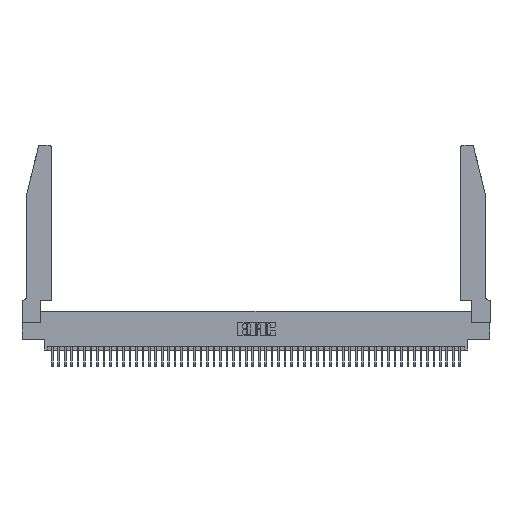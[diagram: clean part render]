
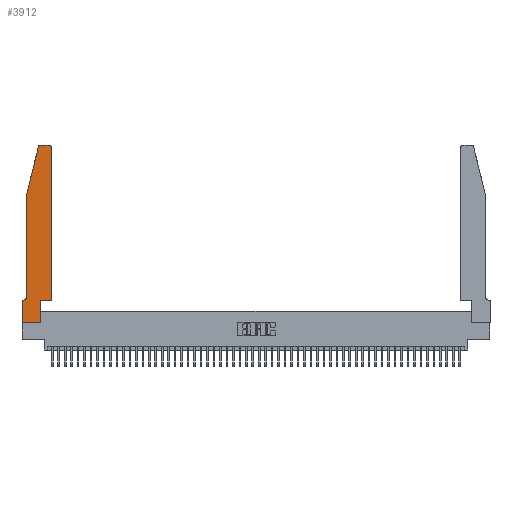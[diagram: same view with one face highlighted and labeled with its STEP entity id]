
A CAD part, top view. The second image highlights one B-rep face of the part: STEP entity #3912.
In plain terms, the highlighted planar face has unit normal (0, 0, 1).
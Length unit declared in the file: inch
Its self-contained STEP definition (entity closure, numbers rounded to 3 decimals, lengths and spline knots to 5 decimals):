
#537 = DIRECTION ( 'NONE',  ( 0., 0., 1. ) ) ;
#1796 = CARTESIAN_POINT ( 'NONE',  ( 0.4505, 0.35, 0.37 ) ) ;
#2151 = EDGE_CURVE ( 'NONE', #37562, #42521, #5699, .T. ) ;
#2193 = LINE ( 'NONE', #25309, #21605 ) ;
#2784 = VECTOR ( 'NONE', #5472, 39.37008 ) ;
#3248 = ORIENTED_EDGE ( 'NONE', *, *, #9848, .T. ) ;
#3912 = ADVANCED_FACE ( 'NONE', ( #16508 ), #24266, .T. ) ;
#4356 = LINE ( 'NONE', #8426, #35133 ) ;
#4767 = CARTESIAN_POINT ( 'NONE',  ( 0.4505, 0.35, 0.37 ) ) ;
#5472 = DIRECTION ( 'NONE',  ( 0., -1., 0. ) ) ;
#5597 = DIRECTION ( 'NONE',  ( -0.239, -0.971, 0. ) ) ;
#5699 = CIRCLE ( 'NONE', #30577, 0.03 ) ;
#6133 = VERTEX_POINT ( 'NONE', #40541 ) ;
#6648 = AXIS2_PLACEMENT_3D ( 'NONE', #35865, #12809, #39764 ) ;
#6654 = EDGE_CURVE ( 'NONE', #9493, #6133, #28528, .T. ) ;
#7060 = CARTESIAN_POINT ( 'NONE',  ( 0.4505, 0.35, 0.37 ) ) ;
#7397 = CARTESIAN_POINT ( 'NONE',  ( 0.2865, 0.35, 0.37 ) ) ;
#7772 = VECTOR ( 'NONE', #48932, 39.37008 ) ;
#8009 = VECTOR ( 'NONE', #48138, 39.37008 ) ;
#8426 = CARTESIAN_POINT ( 'NONE',  ( 0., 0., 0.37 ) ) ;
#8961 = LINE ( 'NONE', #45038, #7772 ) ;
#9363 = CARTESIAN_POINT ( 'NONE',  ( 0.0755, 2., 0.37 ) ) ;
#9493 = VERTEX_POINT ( 'NONE', #7060 ) ;
#9848 = EDGE_CURVE ( 'NONE', #35684, #33851, #33599, .T. ) ;
#11339 = VERTEX_POINT ( 'NONE', #7397 ) ;
#11398 = LINE ( 'NONE', #32625, #19224 ) ;
#12253 = ORIENTED_EDGE ( 'NONE', *, *, #21079, .T. ) ;
#12809 = DIRECTION ( 'NONE',  ( 0., 0., 1. ) ) ;
#12898 = EDGE_CURVE ( 'NONE', #11339, #9493, #33223, .T. ) ;
#13125 = LINE ( 'NONE', #45137, #33621 ) ;
#14284 = EDGE_CURVE ( 'NONE', #43048, #31993, #29478, .T. ) ;
#16508 = FACE_OUTER_BOUND ( 'NONE', #26157, .T. ) ;
#17148 = CIRCLE ( 'NONE', #38379, 0.03 ) ;
#17842 = EDGE_CURVE ( 'NONE', #19647, #37562, #13125, .T. ) ;
#18845 = VERTEX_POINT ( 'NONE', #43489 ) ;
#19224 = VECTOR ( 'NONE', #5597, 39.37008 ) ;
#19528 = CARTESIAN_POINT ( 'NONE',  ( 0.284, 2.75, 0.37 ) ) ;
#19647 = VERTEX_POINT ( 'NONE', #49187 ) ;
#20992 = VERTEX_POINT ( 'NONE', #44925 ) ;
#21079 = EDGE_CURVE ( 'NONE', #33851, #18845, #48440, .T. ) ;
#21605 = VECTOR ( 'NONE', #29178, 39.37008 ) ;
#22014 = DIRECTION ( 'NONE',  ( -1., 0., 0. ) ) ;
#22317 = CARTESIAN_POINT ( 'NONE',  ( 0.0055, 0.42, 0.37 ) ) ;
#22458 = ORIENTED_EDGE ( 'NONE', *, *, #17842, .T. ) ;
#23004 = CARTESIAN_POINT ( 'NONE',  ( 0.4205, 2.72, 0.37 ) ) ;
#23778 = CARTESIAN_POINT ( 'NONE',  ( 0.284, 2.72, 0.37 ) ) ;
#24104 = EDGE_CURVE ( 'NONE', #18845, #20992, #2193, .T. ) ;
#24266 = PLANE ( 'NONE',  #6648 ) ;
#25067 = ORIENTED_EDGE ( 'NONE', *, *, #6654, .T. ) ;
#25309 = CARTESIAN_POINT ( 'NONE',  ( 0.0755, 0.35, 0.37 ) ) ;
#25666 = CARTESIAN_POINT ( 'NONE',  ( 0.0755, 0.42, 0.37 ) ) ;
#25700 = ORIENTED_EDGE ( 'NONE', *, *, #12898, .T. ) ;
#26157 = EDGE_LOOP ( 'NONE', ( #22458, #41080, #29340, #3248, #12253, #31574, #48943, #39604, #47365, #25700, #25067, #43212 ) ) ;
#26176 = DIRECTION ( 'NONE',  ( -1., 0., 0. ) ) ;
#26900 = DIRECTION ( 'NONE',  ( 1., 0., 0. ) ) ;
#27680 = DIRECTION ( 'NONE',  ( 1., 0., 0. ) ) ;
#28528 = LINE ( 'NONE', #1796, #8009 ) ;
#29178 = DIRECTION ( 'NONE',  ( -1., 0., 0. ) ) ;
#29340 = ORIENTED_EDGE ( 'NONE', *, *, #47243, .T. ) ;
#29478 = LINE ( 'NONE', #40960, #48831 ) ;
#30577 = AXIS2_PLACEMENT_3D ( 'NONE', #23778, #537, #27680 ) ;
#30876 = EDGE_CURVE ( 'NONE', #6133, #19647, #17148, .T. ) ;
#31273 = CARTESIAN_POINT ( 'NONE',  ( 0.25487, 2.72718, 0.37 ) ) ;
#31574 = ORIENTED_EDGE ( 'NONE', *, *, #24104, .T. ) ;
#31993 = VERTEX_POINT ( 'NONE', #44660 ) ;
#32019 = VECTOR ( 'NONE', #47167, 39.37008 ) ;
#32625 = CARTESIAN_POINT ( 'NONE',  ( 0.0755, 2., 0.37 ) ) ;
#33223 = LINE ( 'NONE', #4767, #32019 ) ;
#33599 = LINE ( 'NONE', #9363, #2784 ) ;
#33621 = VECTOR ( 'NONE', #22014, 39.37008 ) ;
#33851 = VERTEX_POINT ( 'NONE', #25666 ) ;
#35133 = VECTOR ( 'NONE', #35390, 39.37008 ) ;
#35390 = DIRECTION ( 'NONE',  ( 0., -1., 0. ) ) ;
#35505 = EDGE_CURVE ( 'NONE', #31993, #11339, #8961, .T. ) ;
#35684 = VERTEX_POINT ( 'NONE', #38235 ) ;
#35865 = CARTESIAN_POINT ( 'NONE',  ( 0., 0.35, 0.37 ) ) ;
#37562 = VERTEX_POINT ( 'NONE', #19528 ) ;
#38108 = CARTESIAN_POINT ( 'NONE',  ( 0., 0., 0.37 ) ) ;
#38235 = CARTESIAN_POINT ( 'NONE',  ( 0.0755, 2., 0.37 ) ) ;
#38379 = AXIS2_PLACEMENT_3D ( 'NONE', #23004, #50022, #26900 ) ;
#39512 = EDGE_CURVE ( 'NONE', #20992, #43048, #4356, .T. ) ;
#39604 = ORIENTED_EDGE ( 'NONE', *, *, #14284, .T. ) ;
#39764 = DIRECTION ( 'NONE',  ( 1., 0., 0. ) ) ;
#40541 = CARTESIAN_POINT ( 'NONE',  ( 0.4505, 2.72, 0.37 ) ) ;
#40960 = CARTESIAN_POINT ( 'NONE',  ( 0., 0., 0.37 ) ) ;
#41080 = ORIENTED_EDGE ( 'NONE', *, *, #2151, .T. ) ;
#42521 = VERTEX_POINT ( 'NONE', #31273 ) ;
#43048 = VERTEX_POINT ( 'NONE', #38108 ) ;
#43212 = ORIENTED_EDGE ( 'NONE', *, *, #30876, .T. ) ;
#43489 = CARTESIAN_POINT ( 'NONE',  ( 0.0055, 0.35, 0.37 ) ) ;
#44660 = CARTESIAN_POINT ( 'NONE',  ( 0.2865, 0., 0.37 ) ) ;
#44925 = CARTESIAN_POINT ( 'NONE',  ( 0., 0.35, 0.37 ) ) ;
#45038 = CARTESIAN_POINT ( 'NONE',  ( 0.2865, 0.35, 0.37 ) ) ;
#45137 = CARTESIAN_POINT ( 'NONE',  ( 0.2605, 2.75, 0.37 ) ) ;
#45273 = AXIS2_PLACEMENT_3D ( 'NONE', #22317, #49317, #26176 ) ;
#47167 = DIRECTION ( 'NONE',  ( 1., 0., 0. ) ) ;
#47243 = EDGE_CURVE ( 'NONE', #42521, #35684, #11398, .T. ) ;
#47365 = ORIENTED_EDGE ( 'NONE', *, *, #35505, .T. ) ;
#48138 = DIRECTION ( 'NONE',  ( 0., 1., 0. ) ) ;
#48440 = CIRCLE ( 'NONE', #45273, 0.07 ) ;
#48763 = DIRECTION ( 'NONE',  ( 1., 0., 0. ) ) ;
#48831 = VECTOR ( 'NONE', #48763, 39.37008 ) ;
#48932 = DIRECTION ( 'NONE',  ( 0., 1., 0. ) ) ;
#48943 = ORIENTED_EDGE ( 'NONE', *, *, #39512, .T. ) ;
#49187 = CARTESIAN_POINT ( 'NONE',  ( 0.4205, 2.75, 0.37 ) ) ;
#49317 = DIRECTION ( 'NONE',  ( 0., 0., -1. ) ) ;
#50022 = DIRECTION ( 'NONE',  ( 0., 0., 1. ) ) ;
